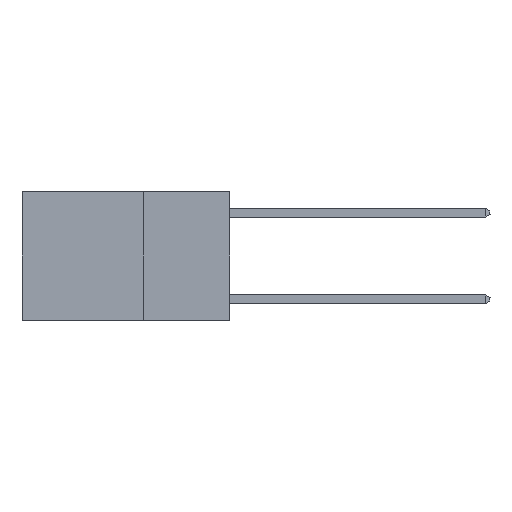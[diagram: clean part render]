
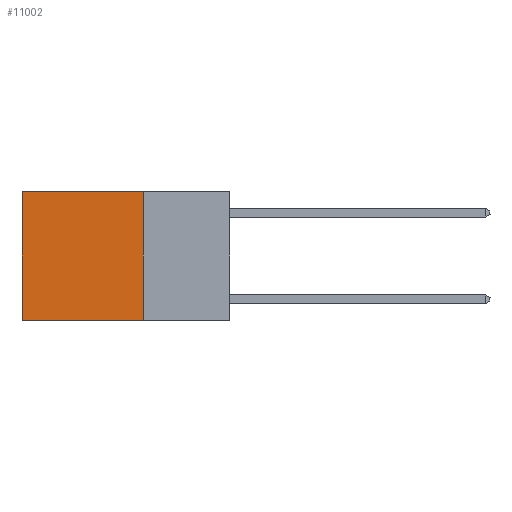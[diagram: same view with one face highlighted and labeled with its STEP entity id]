
A CAD part, left-side view. The second image highlights one B-rep face of the part: STEP entity #11002.
In plain terms, the highlighted planar face has unit normal (-1, 0, 0).
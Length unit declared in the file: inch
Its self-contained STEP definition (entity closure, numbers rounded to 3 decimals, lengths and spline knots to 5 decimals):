
#289 = DIRECTION ( 'NONE',  ( 0., 0., -1. ) ) ;
#1008 = CARTESIAN_POINT ( 'NONE',  ( 0.2625, 0.25, 0. ) ) ;
#1541 = VECTOR ( 'NONE', #8227, 39.37008 ) ;
#1616 = CARTESIAN_POINT ( 'NONE',  ( 0.2625, 0.6, 0. ) ) ;
#1721 = ORIENTED_EDGE ( 'NONE', *, *, #15160, .F. ) ;
#1775 = ORIENTED_EDGE ( 'NONE', *, *, #14537, .F. ) ;
#2132 = EDGE_LOOP ( 'NONE', ( #10165, #1775, #1721, #11382 ) ) ;
#2383 = VERTEX_POINT ( 'NONE', #1616 ) ;
#2708 = CARTESIAN_POINT ( 'NONE',  ( 0.2625, 0.25, 0. ) ) ;
#3762 = CARTESIAN_POINT ( 'NONE',  ( 0.2625, 0.6, 0. ) ) ;
#3858 = CARTESIAN_POINT ( 'NONE',  ( 0.2625, 0.6, -0.37 ) ) ;
#6575 = CARTESIAN_POINT ( 'NONE',  ( 0.2625, 0.25, -0.37 ) ) ;
#6677 = LINE ( 'NONE', #2708, #1541 ) ;
#8227 = DIRECTION ( 'NONE',  ( 0., 1., 0. ) ) ;
#8575 = VECTOR ( 'NONE', #19702, 39.37008 ) ;
#9105 = VERTEX_POINT ( 'NONE', #3858 ) ;
#10165 = ORIENTED_EDGE ( 'NONE', *, *, #17484, .T. ) ;
#10235 = PLANE ( 'NONE',  #20270 ) ;
#10337 = EDGE_CURVE ( 'NONE', #23449, #2383, #6677, .T. ) ;
#11002 = ADVANCED_FACE ( 'NONE', ( #21072 ), #10235, .F. ) ;
#11382 = ORIENTED_EDGE ( 'NONE', *, *, #10337, .T. ) ;
#11448 = LINE ( 'NONE', #3762, #14979 ) ;
#11928 = DIRECTION ( 'NONE',  ( 0., 0., -1. ) ) ;
#12231 = DIRECTION ( 'NONE',  ( 0., 1., 0. ) ) ;
#12381 = CARTESIAN_POINT ( 'NONE',  ( 0.2625, 0.25, 0. ) ) ;
#13942 = CARTESIAN_POINT ( 'NONE',  ( 0.2625, 0.25, 0. ) ) ;
#14537 = EDGE_CURVE ( 'NONE', #17369, #9105, #21134, .T. ) ;
#14979 = VECTOR ( 'NONE', #289, 39.37008 ) ;
#15160 = EDGE_CURVE ( 'NONE', #23449, #17369, #21511, .T. ) ;
#17369 = VERTEX_POINT ( 'NONE', #6575 ) ;
#17484 = EDGE_CURVE ( 'NONE', #2383, #9105, #11448, .T. ) ;
#18146 = VECTOR ( 'NONE', #12231, 39.37008 ) ;
#19702 = DIRECTION ( 'NONE',  ( 0., 0., -1. ) ) ;
#20270 = AXIS2_PLACEMENT_3D ( 'NONE', #1008, #23358, #11928 ) ;
#21028 = CARTESIAN_POINT ( 'NONE',  ( 0.2625, 0.25, -0.37 ) ) ;
#21072 = FACE_OUTER_BOUND ( 'NONE', #2132, .T. ) ;
#21134 = LINE ( 'NONE', #21028, #18146 ) ;
#21511 = LINE ( 'NONE', #12381, #8575 ) ;
#23358 = DIRECTION ( 'NONE',  ( 1., 0., 0. ) ) ;
#23449 = VERTEX_POINT ( 'NONE', #13942 ) ;
